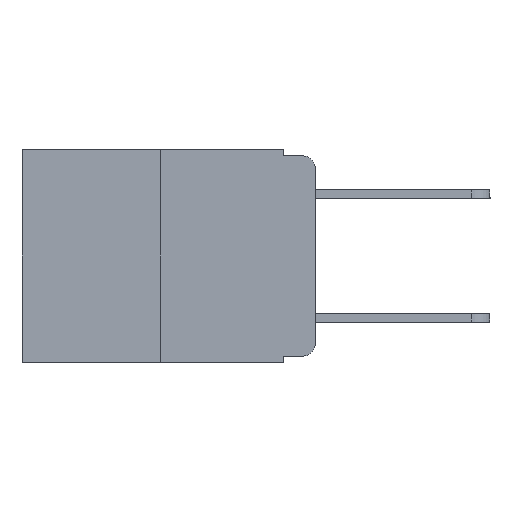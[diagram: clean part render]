
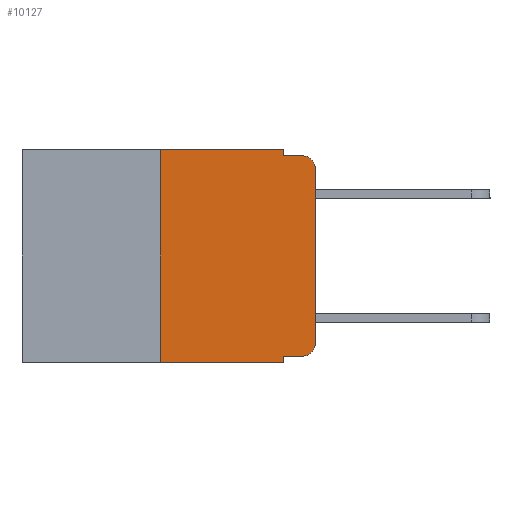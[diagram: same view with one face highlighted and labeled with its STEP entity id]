
A CAD part, left-side view. The second image highlights one B-rep face of the part: STEP entity #10127.
In plain terms, the highlighted planar face has unit normal (-1, 0, 0).
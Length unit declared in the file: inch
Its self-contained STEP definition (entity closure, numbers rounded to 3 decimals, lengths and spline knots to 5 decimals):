
#303 = CARTESIAN_POINT ( 'NONE',  ( 0., 0.051, -0.333 ) ) ;
#466 = CARTESIAN_POINT ( 'NONE',  ( 0., 0.051, 0. ) ) ;
#583 = PLANE ( 'NONE',  #4490 ) ;
#605 = CARTESIAN_POINT ( 'NONE',  ( 0., 0.02, -0.313 ) ) ;
#1246 = VERTEX_POINT ( 'NONE', #16450 ) ;
#1287 = VERTEX_POINT ( 'NONE', #13879 ) ;
#1723 = ORIENTED_EDGE ( 'NONE', *, *, #9530, .F. ) ;
#2048 = VERTEX_POINT ( 'NONE', #10368 ) ;
#2205 = DIRECTION ( 'NONE',  ( 0., 0., -1. ) ) ;
#2213 = VERTEX_POINT ( 'NONE', #8632 ) ;
#2252 = CARTESIAN_POINT ( 'NONE',  ( 0., 0.473, -0.343 ) ) ;
#2452 = LINE ( 'NONE', #466, #16263 ) ;
#2768 = LINE ( 'NONE', #2942, #16489 ) ;
#2942 = CARTESIAN_POINT ( 'NONE',  ( 0., 0.473, 0. ) ) ;
#3688 = CARTESIAN_POINT ( 'NONE',  ( 0., 0.473, 0. ) ) ;
#4116 = ORIENTED_EDGE ( 'NONE', *, *, #11040, .F. ) ;
#4359 = ORIENTED_EDGE ( 'NONE', *, *, #11041, .T. ) ;
#4490 = AXIS2_PLACEMENT_3D ( 'NONE', #3688, #8137, #16813 ) ;
#5232 = CARTESIAN_POINT ( 'NONE',  ( 0., 0.051, -0.333 ) ) ;
#5628 = VECTOR ( 'NONE', #12211, 39.37008 ) ;
#5946 = CARTESIAN_POINT ( 'NONE',  ( 0., 0.02, -0.03 ) ) ;
#6036 = VERTEX_POINT ( 'NONE', #303 ) ;
#6037 = ORIENTED_EDGE ( 'NONE', *, *, #10128, .T. ) ;
#6602 = DIRECTION ( 'NONE',  ( 0., 0., -1. ) ) ;
#6670 = DIRECTION ( 'NONE',  ( 0., -1., 0. ) ) ;
#7190 = VERTEX_POINT ( 'NONE', #16193 ) ;
#7368 = DIRECTION ( 'NONE',  ( 0., 0., -1. ) ) ;
#7380 = ORIENTED_EDGE ( 'NONE', *, *, #11043, .T. ) ;
#7933 = CARTESIAN_POINT ( 'NONE',  ( 0., 0., -0.03 ) ) ;
#8137 = DIRECTION ( 'NONE',  ( 1., 0., 0. ) ) ;
#8632 = CARTESIAN_POINT ( 'NONE',  ( 0., 0.25, -0.343 ) ) ;
#9284 = CIRCLE ( 'NONE', #15073, 0.02 ) ;
#9400 = ORIENTED_EDGE ( 'NONE', *, *, #11022, .F. ) ;
#9497 = VECTOR ( 'NONE', #12917, 39.37008 ) ;
#9530 = EDGE_CURVE ( 'NONE', #1246, #2048, #2768, .T. ) ;
#9698 = LINE ( 'NONE', #16727, #12802 ) ;
#9989 = VERTEX_POINT ( 'NONE', #10523 ) ;
#10023 = ORIENTED_EDGE ( 'NONE', *, *, #11018, .F. ) ;
#10127 = ADVANCED_FACE ( 'NONE', ( #15227 ), #583, .F. ) ;
#10128 = EDGE_CURVE ( 'NONE', #2213, #1287, #14851, .T. ) ;
#10187 = VECTOR ( 'NONE', #12071, 39.37008 ) ;
#10368 = CARTESIAN_POINT ( 'NONE',  ( 0., 0.051, 0. ) ) ;
#10523 = CARTESIAN_POINT ( 'NONE',  ( 0., 0.02, -0.333 ) ) ;
#10634 = LINE ( 'NONE', #11133, #16605 ) ;
#10764 = EDGE_CURVE ( 'NONE', #13850, #15163, #10634, .T. ) ;
#10864 = EDGE_CURVE ( 'NONE', #15163, #15718, #14822, .T. ) ;
#10882 = DIRECTION ( 'NONE',  ( -1., 0., 0. ) ) ;
#10926 = EDGE_CURVE ( 'NONE', #7190, #15718, #16097, .T. ) ;
#11018 = EDGE_CURVE ( 'NONE', #2048, #7190, #2452, .T. ) ;
#11022 = EDGE_CURVE ( 'NONE', #2213, #1246, #16591, .T. ) ;
#11040 = EDGE_CURVE ( 'NONE', #6036, #1287, #9698, .T. ) ;
#11041 = EDGE_CURVE ( 'NONE', #6036, #9989, #13151, .T. ) ;
#11043 = EDGE_CURVE ( 'NONE', #9989, #13850, #9284, .T. ) ;
#11133 = CARTESIAN_POINT ( 'NONE',  ( 0., 0., 0. ) ) ;
#11825 = CARTESIAN_POINT ( 'NONE',  ( 0., 0., -0.313 ) ) ;
#11828 = ORIENTED_EDGE ( 'NONE', *, *, #10764, .T. ) ;
#11972 = ORIENTED_EDGE ( 'NONE', *, *, #10864, .T. ) ;
#12022 = CARTESIAN_POINT ( 'NONE',  ( 0., 0.02, -0.01 ) ) ;
#12071 = DIRECTION ( 'NONE',  ( 0., 0., 1. ) ) ;
#12211 = DIRECTION ( 'NONE',  ( 0., -1., 0. ) ) ;
#12263 = EDGE_LOOP ( 'NONE', ( #11828, #11972, #14847, #10023, #1723, #9400, #6037, #4116, #4359, #7380 ) ) ;
#12760 = DIRECTION ( 'NONE',  ( 0., -1., 0. ) ) ;
#12802 = VECTOR ( 'NONE', #13304, 39.37008 ) ;
#12917 = DIRECTION ( 'NONE',  ( 0., -1., 0. ) ) ;
#13151 = LINE ( 'NONE', #5232, #15914 ) ;
#13304 = DIRECTION ( 'NONE',  ( 0., 0., -1. ) ) ;
#13850 = VERTEX_POINT ( 'NONE', #11825 ) ;
#13879 = CARTESIAN_POINT ( 'NONE',  ( 0., 0.051, -0.343 ) ) ;
#14102 = CARTESIAN_POINT ( 'NONE',  ( 0., 0.051, -0.01 ) ) ;
#14822 = CIRCLE ( 'NONE', #16870, 0.02 ) ;
#14847 = ORIENTED_EDGE ( 'NONE', *, *, #10926, .F. ) ;
#14851 = LINE ( 'NONE', #2252, #5628 ) ;
#15063 = DIRECTION ( 'NONE',  ( -1., 0., 0. ) ) ;
#15073 = AXIS2_PLACEMENT_3D ( 'NONE', #605, #10882, #2205 ) ;
#15163 = VERTEX_POINT ( 'NONE', #7933 ) ;
#15227 = FACE_OUTER_BOUND ( 'NONE', #12263, .T. ) ;
#15621 = CARTESIAN_POINT ( 'NONE',  ( 0., 0.25, 0. ) ) ;
#15718 = VERTEX_POINT ( 'NONE', #12022 ) ;
#15914 = VECTOR ( 'NONE', #6670, 39.37008 ) ;
#16097 = LINE ( 'NONE', #14102, #9497 ) ;
#16193 = CARTESIAN_POINT ( 'NONE',  ( 0., 0.051, -0.01 ) ) ;
#16263 = VECTOR ( 'NONE', #6602, 39.37008 ) ;
#16450 = CARTESIAN_POINT ( 'NONE',  ( 0., 0.25, 0. ) ) ;
#16489 = VECTOR ( 'NONE', #12760, 39.37008 ) ;
#16591 = LINE ( 'NONE', #15621, #10187 ) ;
#16605 = VECTOR ( 'NONE', #16990, 39.37008 ) ;
#16727 = CARTESIAN_POINT ( 'NONE',  ( 0., 0.051, 0. ) ) ;
#16813 = DIRECTION ( 'NONE',  ( 0., 0., -1. ) ) ;
#16870 = AXIS2_PLACEMENT_3D ( 'NONE', #5946, #15063, #7368 ) ;
#16990 = DIRECTION ( 'NONE',  ( 0., 0., 1. ) ) ;
